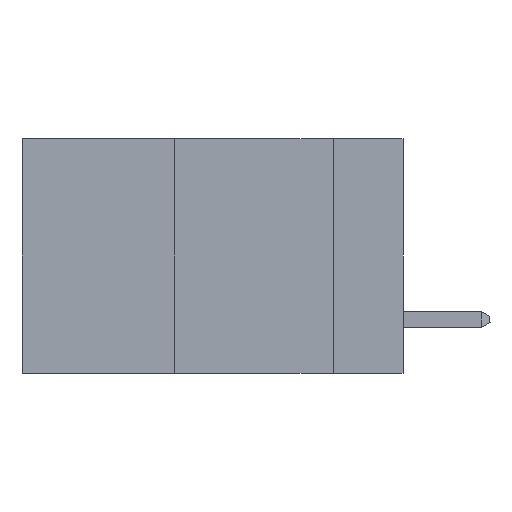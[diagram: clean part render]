
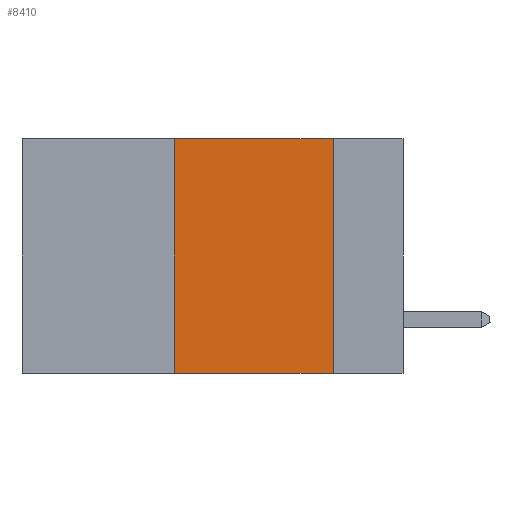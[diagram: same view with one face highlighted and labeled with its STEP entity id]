
A CAD part, left-side view. The second image highlights one B-rep face of the part: STEP entity #8410.
In plain terms, the highlighted planar face has unit normal (-1, 0, 0).
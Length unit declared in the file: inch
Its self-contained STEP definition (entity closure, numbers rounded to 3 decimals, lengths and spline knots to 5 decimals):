
#111 = VECTOR ( 'NONE', #4715, 39.37008 ) ;
#463 = CARTESIAN_POINT ( 'NONE',  ( 0., 0.36, -0.37 ) ) ;
#797 = LINE ( 'NONE', #2498, #111 ) ;
#915 = CARTESIAN_POINT ( 'NONE',  ( 0., 0.11, 0. ) ) ;
#1239 = VECTOR ( 'NONE', #3022, 39.37008 ) ;
#1962 = LINE ( 'NONE', #915, #4953 ) ;
#2335 = EDGE_CURVE ( 'NONE', #3317, #5101, #1962, .T. ) ;
#2498 = CARTESIAN_POINT ( 'NONE',  ( 0., 0.6, 0. ) ) ;
#2706 = PLANE ( 'NONE',  #6404 ) ;
#2891 = CARTESIAN_POINT ( 'NONE',  ( 0., 0.11, -0.37 ) ) ;
#2916 = CARTESIAN_POINT ( 'NONE',  ( 0., 0.11, 0. ) ) ;
#3022 = DIRECTION ( 'NONE',  ( 0., -1., 0. ) ) ;
#3163 = CARTESIAN_POINT ( 'NONE',  ( 0., 0.36, 0. ) ) ;
#3219 = DIRECTION ( 'NONE',  ( 0., 0., -1. ) ) ;
#3317 = VERTEX_POINT ( 'NONE', #2916 ) ;
#3520 = VERTEX_POINT ( 'NONE', #3163 ) ;
#3956 = EDGE_CURVE ( 'NONE', #6654, #3520, #5725, .T. ) ;
#4178 = DIRECTION ( 'NONE',  ( 0., 0., -1. ) ) ;
#4534 = CARTESIAN_POINT ( 'NONE',  ( 0., 0.6, -0.37 ) ) ;
#4715 = DIRECTION ( 'NONE',  ( 0., -1., 0. ) ) ;
#4953 = VECTOR ( 'NONE', #3219, 39.37008 ) ;
#5101 = VERTEX_POINT ( 'NONE', #2891 ) ;
#5176 = ORIENTED_EDGE ( 'NONE', *, *, #3956, .F. ) ;
#5244 = ORIENTED_EDGE ( 'NONE', *, *, #2335, .F. ) ;
#5369 = EDGE_CURVE ( 'NONE', #3520, #3317, #797, .T. ) ;
#5725 = LINE ( 'NONE', #5961, #7544 ) ;
#5954 = LINE ( 'NONE', #4534, #1239 ) ;
#5961 = CARTESIAN_POINT ( 'NONE',  ( 0., 0.36, 0. ) ) ;
#6284 = ORIENTED_EDGE ( 'NONE', *, *, #5369, .F. ) ;
#6404 = AXIS2_PLACEMENT_3D ( 'NONE', #9278, #7762, #4178 ) ;
#6654 = VERTEX_POINT ( 'NONE', #463 ) ;
#6721 = EDGE_LOOP ( 'NONE', ( #5244, #6284, #5176, #6986 ) ) ;
#6937 = EDGE_CURVE ( 'NONE', #6654, #5101, #5954, .T. ) ;
#6986 = ORIENTED_EDGE ( 'NONE', *, *, #6937, .T. ) ;
#7517 = FACE_OUTER_BOUND ( 'NONE', #6721, .T. ) ;
#7544 = VECTOR ( 'NONE', #8141, 39.37008 ) ;
#7762 = DIRECTION ( 'NONE',  ( 1., 0., 0. ) ) ;
#8141 = DIRECTION ( 'NONE',  ( 0., 0., 1. ) ) ;
#8410 = ADVANCED_FACE ( 'NONE', ( #7517 ), #2706, .F. ) ;
#9278 = CARTESIAN_POINT ( 'NONE',  ( 0., 0.6, 0. ) ) ;
